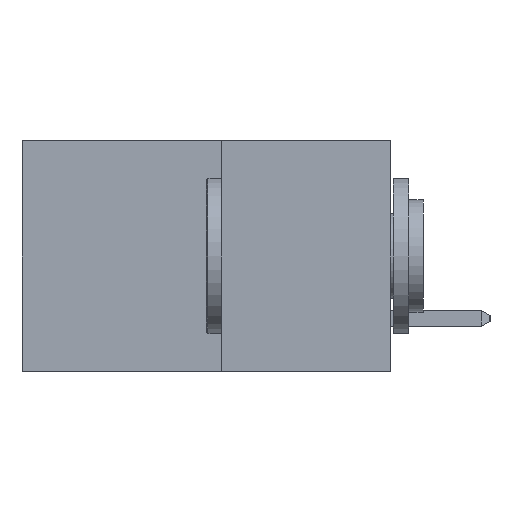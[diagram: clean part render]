
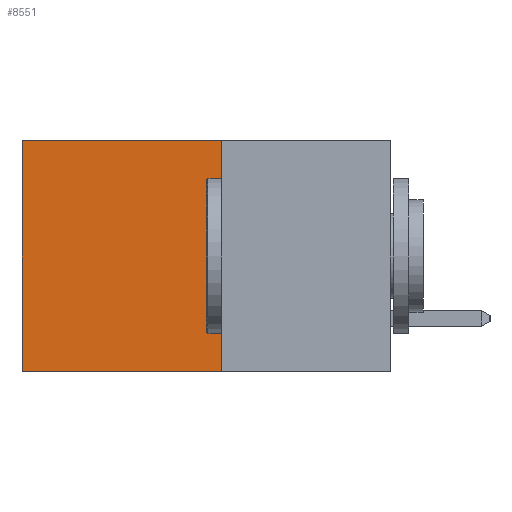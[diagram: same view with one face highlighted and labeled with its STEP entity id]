
A CAD part, left-side view. The second image highlights one B-rep face of the part: STEP entity #8551.
In plain terms, the highlighted planar face has unit normal (-1, 0, 0).
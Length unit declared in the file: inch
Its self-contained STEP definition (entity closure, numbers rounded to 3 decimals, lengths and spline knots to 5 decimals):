
#409 = LINE ( 'NONE', #12867, #10553 ) ;
#874 = DIRECTION ( 'NONE',  ( 0., 1., 0. ) ) ;
#1005 = VECTOR ( 'NONE', #22260, 39.37008 ) ;
#1231 = CARTESIAN_POINT ( 'NONE',  ( 0.277, 0.27, 0. ) ) ;
#1693 = EDGE_CURVE ( 'NONE', #25821, #11831, #7296, .T. ) ;
#1876 = VECTOR ( 'NONE', #21978, 39.37008 ) ;
#2032 = CARTESIAN_POINT ( 'NONE',  ( 0.277, 0.59, -0.37 ) ) ;
#3411 = CARTESIAN_POINT ( 'NONE',  ( 0.277, 0.59, 0. ) ) ;
#4145 = CARTESIAN_POINT ( 'NONE',  ( 0.277, 0.27, -0.37 ) ) ;
#4395 = FACE_OUTER_BOUND ( 'NONE', #8824, .T. ) ;
#5306 = EDGE_CURVE ( 'NONE', #10887, #11831, #7058, .T. ) ;
#5404 = AXIS2_PLACEMENT_3D ( 'NONE', #4145, #18304, #6178 ) ;
#6178 = DIRECTION ( 'NONE',  ( 0., 0., -1. ) ) ;
#6840 = VECTOR ( 'NONE', #874, 39.37008 ) ;
#7058 = LINE ( 'NONE', #10091, #1005 ) ;
#7296 = LINE ( 'NONE', #25472, #1876 ) ;
#8551 = ADVANCED_FACE ( 'NONE', ( #4395 ), #24308, .F. ) ;
#8824 = EDGE_LOOP ( 'NONE', ( #24584, #13415, #23979, #10912 ) ) ;
#10091 = CARTESIAN_POINT ( 'NONE',  ( 0.277, 0.59, -0.37 ) ) ;
#10553 = VECTOR ( 'NONE', #14897, 39.37008 ) ;
#10663 = CARTESIAN_POINT ( 'NONE',  ( 0.277, 0.27, -0.37 ) ) ;
#10887 = VERTEX_POINT ( 'NONE', #3411 ) ;
#10912 = ORIENTED_EDGE ( 'NONE', *, *, #15432, .T. ) ;
#11831 = VERTEX_POINT ( 'NONE', #2032 ) ;
#12066 = VERTEX_POINT ( 'NONE', #1231 ) ;
#12867 = CARTESIAN_POINT ( 'NONE',  ( 0.277, 0.27, -0.37 ) ) ;
#13415 = ORIENTED_EDGE ( 'NONE', *, *, #1693, .F. ) ;
#14897 = DIRECTION ( 'NONE',  ( 0., 0., -1. ) ) ;
#15004 = CARTESIAN_POINT ( 'NONE',  ( 0.277, 0.27, 0. ) ) ;
#15432 = EDGE_CURVE ( 'NONE', #12066, #10887, #18876, .T. ) ;
#18304 = DIRECTION ( 'NONE',  ( 1., 0., 0. ) ) ;
#18876 = LINE ( 'NONE', #15004, #6840 ) ;
#21599 = EDGE_CURVE ( 'NONE', #12066, #25821, #409, .T. ) ;
#21978 = DIRECTION ( 'NONE',  ( 0., 1., 0. ) ) ;
#22260 = DIRECTION ( 'NONE',  ( 0., 0., -1. ) ) ;
#23979 = ORIENTED_EDGE ( 'NONE', *, *, #21599, .F. ) ;
#24308 = PLANE ( 'NONE',  #5404 ) ;
#24584 = ORIENTED_EDGE ( 'NONE', *, *, #5306, .T. ) ;
#25472 = CARTESIAN_POINT ( 'NONE',  ( 0.277, 0.27, -0.37 ) ) ;
#25821 = VERTEX_POINT ( 'NONE', #10663 ) ;
